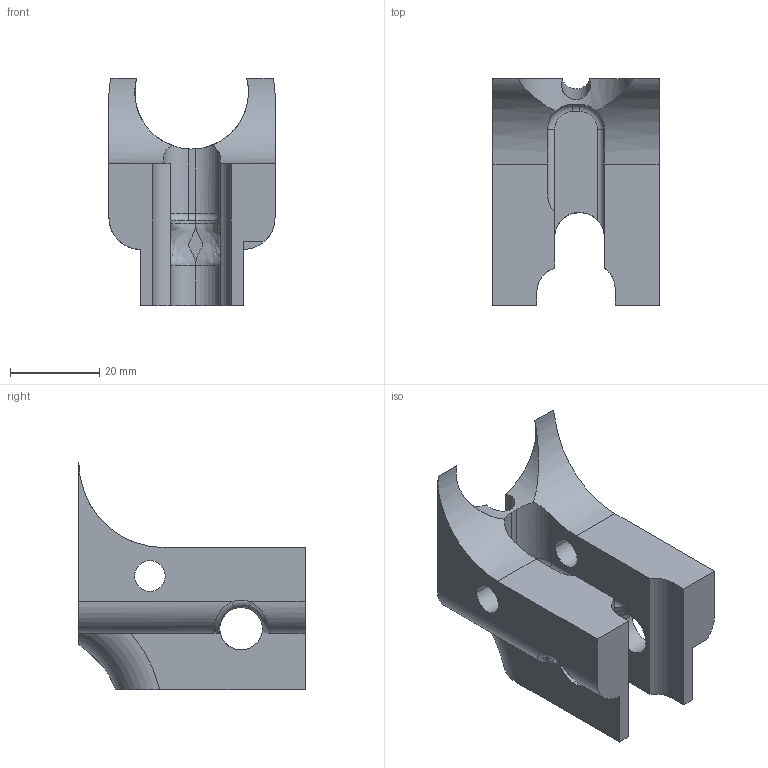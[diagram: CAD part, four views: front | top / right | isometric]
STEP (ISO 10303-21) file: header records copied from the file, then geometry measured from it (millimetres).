
FILE_DESCRIPTION (( 'STEP AP214' ), '1' );
FILE_NAME ('5.STEP', '2013-09-29T07:11:00', ( 'elpi' ), ( '' ), 'SwSTEP 2.0', 'SolidWorks 2013', '' );
FILE_SCHEMA (( 'AUTOMOTIVE_DESIGN' ));
Length unit declared in the file: millimetre
Products named in the file (1): 5
Bounding box: 37.13 x 50.59 x 50.8 mm (x, y, z)
Volume: 33792.1 mm3; surface area: 11049.7 mm2
Topology: 1 solids, 1 shells, 77 faces, 231 edges, 153 vertices
Faces by surface type: cylinder 39, plane 25, bspline 8, torus 5
Entity records: 4321 total; most frequent: CARTESIAN_POINT 2289, ORIENTED_EDGE 462, DIRECTION 371, EDGE_CURVE 231, VERTEX_POINT 153, AXIS2_PLACEMENT_3D 135, LINE 101, VECTOR 101
